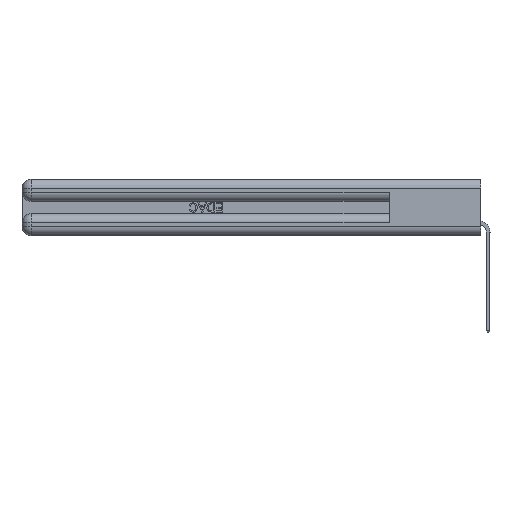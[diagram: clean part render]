
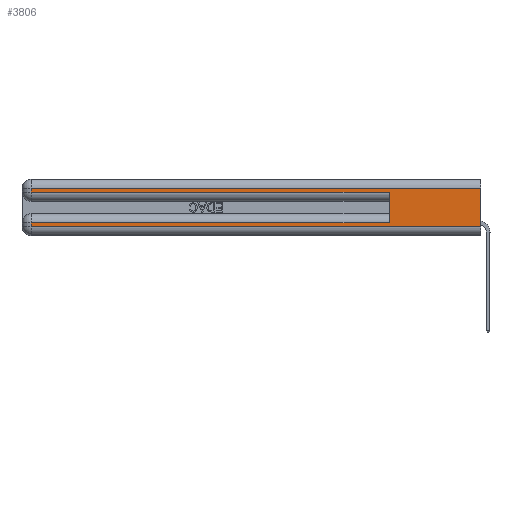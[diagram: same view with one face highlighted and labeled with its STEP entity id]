
A CAD part, left-side view. The second image highlights one B-rep face of the part: STEP entity #3806.
In plain terms, the highlighted planar face has unit normal (-1, 0, 0).
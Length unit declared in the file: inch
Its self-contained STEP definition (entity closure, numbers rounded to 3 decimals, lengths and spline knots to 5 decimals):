
#547 = CARTESIAN_POINT ( 'NONE',  ( 0., 0., 0.085 ) ) ;
#1239 = DIRECTION ( 'NONE',  ( 0., 1., 0. ) ) ;
#1728 = DIRECTION ( 'NONE',  ( 0., -1., 0. ) ) ;
#2340 = CARTESIAN_POINT ( 'NONE',  ( 0., 2.94, 0.06 ) ) ;
#2464 = LINE ( 'NONE', #4939, #15907 ) ;
#3267 = ORIENTED_EDGE ( 'NONE', *, *, #20714, .T. ) ;
#3277 = LINE ( 'NONE', #46380, #17272 ) ;
#3806 = ADVANCED_FACE ( 'NONE', ( #21788 ), #29740, .F. ) ;
#4939 = CARTESIAN_POINT ( 'NONE',  ( 0., 0., 0.31 ) ) ;
#5333 = CARTESIAN_POINT ( 'NONE',  ( 0., 2.94, 0.285 ) ) ;
#5691 = VECTOR ( 'NONE', #37273, 39.37008 ) ;
#9684 = EDGE_CURVE ( 'NONE', #12099, #39801, #3277, .T. ) ;
#9963 = DIRECTION ( 'NONE',  ( 0., 0., -1. ) ) ;
#11373 = VECTOR ( 'NONE', #9963, 39.37008 ) ;
#12099 = VERTEX_POINT ( 'NONE', #17730 ) ;
#12347 = CARTESIAN_POINT ( 'NONE',  ( 0., 0., 0.285 ) ) ;
#12516 = CARTESIAN_POINT ( 'NONE',  ( 0., 2.94, 0.085 ) ) ;
#12594 = VERTEX_POINT ( 'NONE', #43642 ) ;
#12893 = LINE ( 'NONE', #21207, #30923 ) ;
#13332 = VECTOR ( 'NONE', #41072, 39.37008 ) ;
#13891 = LINE ( 'NONE', #12347, #22220 ) ;
#14589 = EDGE_CURVE ( 'NONE', #32401, #12099, #2464, .T. ) ;
#15419 = EDGE_CURVE ( 'NONE', #24382, #42255, #32254, .T. ) ;
#15721 = CARTESIAN_POINT ( 'NONE',  ( 0., 0., 0.06 ) ) ;
#15907 = VECTOR ( 'NONE', #1239, 39.37008 ) ;
#16419 = VECTOR ( 'NONE', #21096, 39.37008 ) ;
#16634 = ORIENTED_EDGE ( 'NONE', *, *, #28505, .F. ) ;
#17272 = VECTOR ( 'NONE', #28543, 39.37008 ) ;
#17730 = CARTESIAN_POINT ( 'NONE',  ( 0., 2.94, 0.31 ) ) ;
#20714 = EDGE_CURVE ( 'NONE', #39801, #32706, #13891, .T. ) ;
#20826 = VERTEX_POINT ( 'NONE', #12516 ) ;
#20985 = LINE ( 'NONE', #42047, #11373 ) ;
#21096 = DIRECTION ( 'NONE',  ( 0., -1., 0. ) ) ;
#21207 = CARTESIAN_POINT ( 'NONE',  ( 0., 0.6, 0.145 ) ) ;
#21788 = FACE_OUTER_BOUND ( 'NONE', #36694, .T. ) ;
#22107 = ORIENTED_EDGE ( 'NONE', *, *, #42529, .F. ) ;
#22220 = VECTOR ( 'NONE', #1728, 39.37008 ) ;
#22944 = CARTESIAN_POINT ( 'NONE',  ( 0., 0., 0.37 ) ) ;
#23162 = CARTESIAN_POINT ( 'NONE',  ( 0., 2.94, 0.37 ) ) ;
#24382 = VERTEX_POINT ( 'NONE', #2340 ) ;
#24723 = CARTESIAN_POINT ( 'NONE',  ( 0., 0., 0.31 ) ) ;
#25905 = LINE ( 'NONE', #547, #5691 ) ;
#26956 = EDGE_CURVE ( 'NONE', #12594, #20826, #25905, .T. ) ;
#27588 = DIRECTION ( 'NONE',  ( 1., 0., 0. ) ) ;
#28505 = EDGE_CURVE ( 'NONE', #12594, #32706, #12893, .T. ) ;
#28543 = DIRECTION ( 'NONE',  ( 0., 0., -1. ) ) ;
#29740 = PLANE ( 'NONE',  #35743 ) ;
#30923 = VECTOR ( 'NONE', #46476, 39.37008 ) ;
#31402 = EDGE_CURVE ( 'NONE', #20826, #24382, #44302, .T. ) ;
#32254 = LINE ( 'NONE', #39489, #16419 ) ;
#32401 = VERTEX_POINT ( 'NONE', #24723 ) ;
#32706 = VERTEX_POINT ( 'NONE', #44383 ) ;
#34563 = DIRECTION ( 'NONE',  ( 0., 0., -1. ) ) ;
#35743 = AXIS2_PLACEMENT_3D ( 'NONE', #22944, #27588, #34563 ) ;
#36694 = EDGE_LOOP ( 'NONE', ( #22107, #44638, #37854, #3267, #16634, #39921, #43535, #44375 ) ) ;
#37273 = DIRECTION ( 'NONE',  ( 0., 1., 0. ) ) ;
#37854 = ORIENTED_EDGE ( 'NONE', *, *, #9684, .T. ) ;
#39489 = CARTESIAN_POINT ( 'NONE',  ( 0., 0., 0.06 ) ) ;
#39801 = VERTEX_POINT ( 'NONE', #5333 ) ;
#39921 = ORIENTED_EDGE ( 'NONE', *, *, #26956, .T. ) ;
#41072 = DIRECTION ( 'NONE',  ( 0., 0., -1. ) ) ;
#42047 = CARTESIAN_POINT ( 'NONE',  ( 0., 0., 0.37 ) ) ;
#42255 = VERTEX_POINT ( 'NONE', #15721 ) ;
#42529 = EDGE_CURVE ( 'NONE', #32401, #42255, #20985, .T. ) ;
#43535 = ORIENTED_EDGE ( 'NONE', *, *, #31402, .T. ) ;
#43642 = CARTESIAN_POINT ( 'NONE',  ( 0., 0.6, 0.085 ) ) ;
#44302 = LINE ( 'NONE', #23162, #13332 ) ;
#44375 = ORIENTED_EDGE ( 'NONE', *, *, #15419, .T. ) ;
#44383 = CARTESIAN_POINT ( 'NONE',  ( 0., 0.6, 0.285 ) ) ;
#44638 = ORIENTED_EDGE ( 'NONE', *, *, #14589, .T. ) ;
#46380 = CARTESIAN_POINT ( 'NONE',  ( 0., 2.94, 0.37 ) ) ;
#46476 = DIRECTION ( 'NONE',  ( 0., 0., 1. ) ) ;
